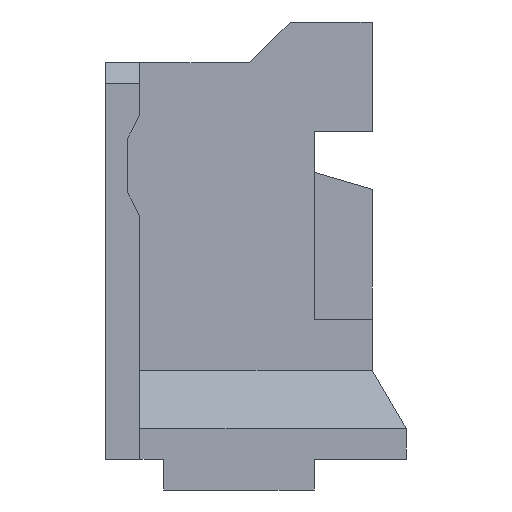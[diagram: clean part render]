
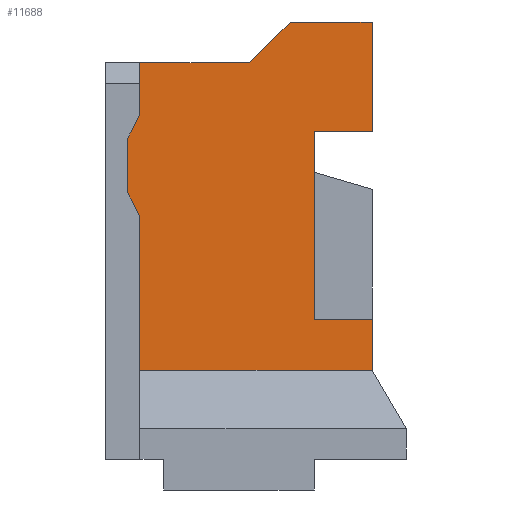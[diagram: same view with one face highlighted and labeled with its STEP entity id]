
A CAD part, left-side view. The second image highlights one B-rep face of the part: STEP entity #11688.
In plain terms, the highlighted planar face has unit normal (-1, 0, 0).
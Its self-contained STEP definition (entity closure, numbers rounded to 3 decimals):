
#145 = ORIENTED_EDGE ( 'NONE', *, *, #12974, .F. ) ;
#216 = VERTEX_POINT ( 'NONE', #9074 ) ;
#292 = CARTESIAN_POINT ( 'NONE',  ( -1.25, 1.1, -5.8 ) ) ;
#394 = VERTEX_POINT ( 'NONE', #11768 ) ;
#467 = EDGE_CURVE ( 'NONE', #12666, #8685, #2969, .T. ) ;
#640 = VECTOR ( 'NONE', #4013, 1000. ) ;
#843 = CARTESIAN_POINT ( 'NONE',  ( -1.25, -1.45, -3.75 ) ) ;
#854 = CARTESIAN_POINT ( 'NONE',  ( -1.25, 1.1, -0.75 ) ) ;
#915 = ORIENTED_EDGE ( 'NONE', *, *, #12391, .F. ) ;
#952 = ORIENTED_EDGE ( 'NONE', *, *, #5523, .F. ) ;
#957 = ORIENTED_EDGE ( 'NONE', *, *, #14370, .F. ) ;
#974 = CARTESIAN_POINT ( 'NONE',  ( -1.25, -2.3, -1.85 ) ) ;
#982 = EDGE_CURVE ( 'NONE', #2504, #13208, #4260, .T. ) ;
#1644 = EDGE_CURVE ( 'NONE', #15226, #394, #2562, .T. ) ;
#1688 = ORIENTED_EDGE ( 'NONE', *, *, #12799, .F. ) ;
#1774 = CARTESIAN_POINT ( 'NONE',  ( -1.25, -1.1, 0.6 ) ) ;
#1843 = CARTESIAN_POINT ( 'NONE',  ( -1.25, -2.3, -1. ) ) ;
#1928 = LINE ( 'NONE', #1843, #12145 ) ;
#2202 = DIRECTION ( 'NONE',  ( 0., 0., -1. ) ) ;
#2440 = CARTESIAN_POINT ( 'NONE',  ( -1.25, -1.45, -1. ) ) ;
#2504 = VERTEX_POINT ( 'NONE', #6500 ) ;
#2551 = DIRECTION ( 'NONE',  ( 0., 0., -1. ) ) ;
#2562 = LINE ( 'NONE', #10466, #13505 ) ;
#2676 = DIRECTION ( 'NONE',  ( 0., 0., 1. ) ) ;
#2812 = CARTESIAN_POINT ( 'NONE',  ( -1.25, -0.5, 0. ) ) ;
#2957 = CARTESIAN_POINT ( 'NONE',  ( -1.25, 1.1, -2.25 ) ) ;
#2969 = LINE ( 'NONE', #2440, #3528 ) ;
#3034 = VERTEX_POINT ( 'NONE', #10159 ) ;
#3205 = ORIENTED_EDGE ( 'NONE', *, *, #4978, .F. ) ;
#3528 = VECTOR ( 'NONE', #2551, 1000. ) ;
#3714 = VECTOR ( 'NONE', #11973, 1000. ) ;
#3730 = DIRECTION ( 'NONE',  ( 0., 0., -1. ) ) ;
#3763 = LINE ( 'NONE', #1774, #10432 ) ;
#3867 = VERTEX_POINT ( 'NONE', #8944 ) ;
#3897 = VERTEX_POINT ( 'NONE', #6872 ) ;
#4013 = DIRECTION ( 'NONE',  ( 0., 0., 1. ) ) ;
#4260 = LINE ( 'NONE', #974, #12959 ) ;
#4519 = CARTESIAN_POINT ( 'NONE',  ( -1.25, -2.3, -1. ) ) ;
#4908 = VECTOR ( 'NONE', #8549, 1000. ) ;
#4978 = EDGE_CURVE ( 'NONE', #216, #3034, #6740, .T. ) ;
#5064 = CARTESIAN_POINT ( 'NONE',  ( -1.25, 1.275, -1.1 ) ) ;
#5299 = LINE ( 'NONE', #292, #8255 ) ;
#5321 = DIRECTION ( 'NONE',  ( 0., -1., 0. ) ) ;
#5440 = VECTOR ( 'NONE', #7195, 1000. ) ;
#5523 = EDGE_CURVE ( 'NONE', #3897, #10289, #3763, .T. ) ;
#5777 = ORIENTED_EDGE ( 'NONE', *, *, #9939, .F. ) ;
#6369 = VECTOR ( 'NONE', #14208, 1000. ) ;
#6500 = CARTESIAN_POINT ( 'NONE',  ( -1.25, -2.3, -3.75 ) ) ;
#6707 = DIRECTION ( 'NONE',  ( 0., -0.447, 0.894 ) ) ;
#6720 = FACE_OUTER_BOUND ( 'NONE', #13220, .T. ) ;
#6740 = LINE ( 'NONE', #11980, #4908 ) ;
#6755 = LINE ( 'NONE', #7110, #6369 ) ;
#6811 = ORIENTED_EDGE ( 'NONE', *, *, #10913, .F. ) ;
#6872 = CARTESIAN_POINT ( 'NONE',  ( -1.25, -1.1, 0.6 ) ) ;
#6932 = DIRECTION ( 'NONE',  ( 0., 0.447, 0.894 ) ) ;
#7110 = CARTESIAN_POINT ( 'NONE',  ( -1.25, -3., -4.5 ) ) ;
#7195 = DIRECTION ( 'NONE',  ( 0., -1., 0. ) ) ;
#7690 = ORIENTED_EDGE ( 'NONE', *, *, #1644, .F. ) ;
#7901 = DIRECTION ( 'NONE',  ( 0., 1., 0. ) ) ;
#8188 = ORIENTED_EDGE ( 'NONE', *, *, #467, .F. ) ;
#8255 = VECTOR ( 'NONE', #2676, 1000. ) ;
#8287 = ORIENTED_EDGE ( 'NONE', *, *, #10534, .F. ) ;
#8530 = PLANE ( 'NONE',  #11899 ) ;
#8549 = DIRECTION ( 'NONE',  ( 0., -1., 0. ) ) ;
#8685 = VERTEX_POINT ( 'NONE', #843 ) ;
#8707 = LINE ( 'NONE', #10732, #3714 ) ;
#8726 = VECTOR ( 'NONE', #9755, 1000. ) ;
#8944 = CARTESIAN_POINT ( 'NONE',  ( -1.25, 1.1, -4.5 ) ) ;
#9074 = CARTESIAN_POINT ( 'NONE',  ( -1.25, 1.1, 0. ) ) ;
#9265 = CARTESIAN_POINT ( 'NONE',  ( -1.25, 1.1, -5.8 ) ) ;
#9323 = LINE ( 'NONE', #10127, #10833 ) ;
#9354 = CARTESIAN_POINT ( 'NONE',  ( -1.25, 3.057, -3.75 ) ) ;
#9755 = DIRECTION ( 'NONE',  ( 0., -0.707, 0.707 ) ) ;
#9929 = CARTESIAN_POINT ( 'NONE',  ( -1.25, -2.3, 0.6 ) ) ;
#9939 = EDGE_CURVE ( 'NONE', #12653, #12666, #1928, .T. ) ;
#10127 = CARTESIAN_POINT ( 'NONE',  ( -1.25, 1.1, -0.75 ) ) ;
#10159 = CARTESIAN_POINT ( 'NONE',  ( -1.25, -0.5, 0. ) ) ;
#10195 = CARTESIAN_POINT ( 'NONE',  ( -1.25, -2.3, -4.5 ) ) ;
#10289 = VERTEX_POINT ( 'NONE', #9929 ) ;
#10374 = VECTOR ( 'NONE', #14094, 1000. ) ;
#10432 = VECTOR ( 'NONE', #5321, 1000. ) ;
#10466 = CARTESIAN_POINT ( 'NONE',  ( -1.25, 1.1, -2.25 ) ) ;
#10534 = EDGE_CURVE ( 'NONE', #14421, #14604, #9323, .T. ) ;
#10732 = CARTESIAN_POINT ( 'NONE',  ( -1.25, -2.3, 0.6 ) ) ;
#10833 = VECTOR ( 'NONE', #6707, 1000. ) ;
#10913 = EDGE_CURVE ( 'NONE', #13208, #3867, #6755, .T. ) ;
#11473 = ORIENTED_EDGE ( 'NONE', *, *, #11545, .F. ) ;
#11490 = ORIENTED_EDGE ( 'NONE', *, *, #982, .F. ) ;
#11545 = EDGE_CURVE ( 'NONE', #8685, #2504, #13950, .T. ) ;
#11688 = ADVANCED_FACE ( 'NONE', ( #6720 ), #8530, .F. ) ;
#11768 = CARTESIAN_POINT ( 'NONE',  ( -1.25, 1.275, -1.9 ) ) ;
#11899 = AXIS2_PLACEMENT_3D ( 'NONE', #12107, #14546, #3730 ) ;
#11973 = DIRECTION ( 'NONE',  ( 0., 0., -1. ) ) ;
#11980 = CARTESIAN_POINT ( 'NONE',  ( -1.25, 1.1, 0. ) ) ;
#12107 = CARTESIAN_POINT ( 'NONE',  ( -1.25, 0., 0. ) ) ;
#12145 = VECTOR ( 'NONE', #7901, 1000. ) ;
#12234 = LINE ( 'NONE', #9265, #10374 ) ;
#12391 = EDGE_CURVE ( 'NONE', #3034, #3897, #12628, .T. ) ;
#12628 = LINE ( 'NONE', #2812, #8726 ) ;
#12653 = VERTEX_POINT ( 'NONE', #4519 ) ;
#12666 = VERTEX_POINT ( 'NONE', #14942 ) ;
#12799 = EDGE_CURVE ( 'NONE', #14604, #216, #12234, .T. ) ;
#12959 = VECTOR ( 'NONE', #2202, 1000. ) ;
#12974 = EDGE_CURVE ( 'NONE', #10289, #12653, #8707, .T. ) ;
#13208 = VERTEX_POINT ( 'NONE', #10195 ) ;
#13220 = EDGE_LOOP ( 'NONE', ( #1688, #8287, #14105, #7690, #957, #6811, #11490, #11473, #8188, #5777, #145, #952, #915, #3205 ) ) ;
#13505 = VECTOR ( 'NONE', #6932, 1000. ) ;
#13950 = LINE ( 'NONE', #9354, #5440 ) ;
#14094 = DIRECTION ( 'NONE',  ( 0., 0., 1. ) ) ;
#14105 = ORIENTED_EDGE ( 'NONE', *, *, #15071, .F. ) ;
#14208 = DIRECTION ( 'NONE',  ( 0., 1., 0. ) ) ;
#14370 = EDGE_CURVE ( 'NONE', #3867, #15226, #5299, .T. ) ;
#14421 = VERTEX_POINT ( 'NONE', #5064 ) ;
#14546 = DIRECTION ( 'NONE',  ( 1., 0., 0. ) ) ;
#14576 = CARTESIAN_POINT ( 'NONE',  ( -1.25, 1.275, -2.25 ) ) ;
#14604 = VERTEX_POINT ( 'NONE', #854 ) ;
#14942 = CARTESIAN_POINT ( 'NONE',  ( -1.25, -1.45, -1. ) ) ;
#15071 = EDGE_CURVE ( 'NONE', #394, #14421, #15122, .T. ) ;
#15122 = LINE ( 'NONE', #14576, #640 ) ;
#15226 = VERTEX_POINT ( 'NONE', #2957 ) ;
